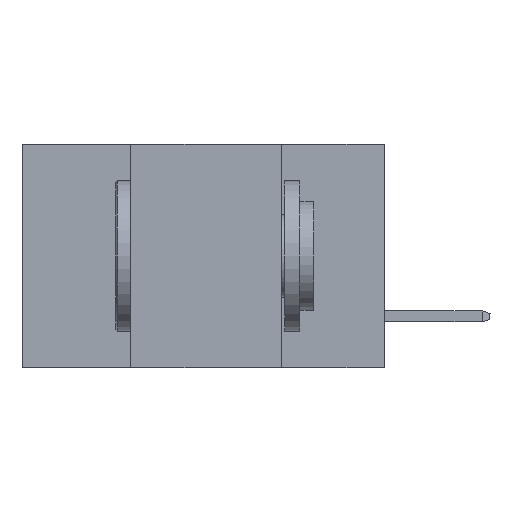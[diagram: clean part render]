
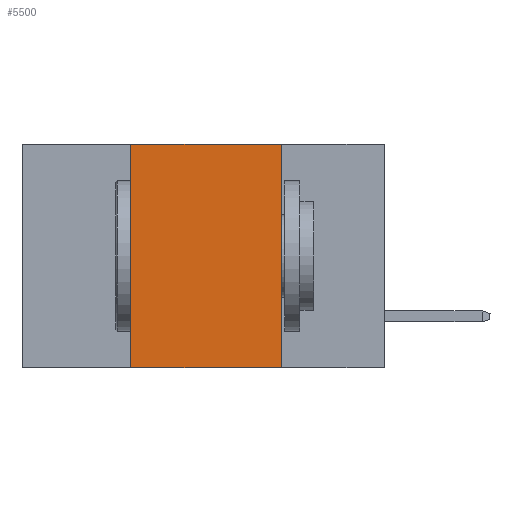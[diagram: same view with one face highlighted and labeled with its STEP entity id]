
A CAD part, left-side view. The second image highlights one B-rep face of the part: STEP entity #5500.
In plain terms, the highlighted planar face has unit normal (-1, 0, 0).
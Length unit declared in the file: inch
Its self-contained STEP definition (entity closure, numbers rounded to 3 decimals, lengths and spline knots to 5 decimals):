
#120 = VECTOR ( 'NONE', #9460, 39.37008 ) ;
#248 = ORIENTED_EDGE ( 'NONE', *, *, #519, .F. ) ;
#519 = EDGE_CURVE ( 'NONE', #4110, #1540, #8587, .T. ) ;
#628 = VECTOR ( 'NONE', #6161, 39.37008 ) ;
#890 = VECTOR ( 'NONE', #1525, 39.37008 ) ;
#1060 = CARTESIAN_POINT ( 'NONE',  ( 0., 0.6, 0. ) ) ;
#1525 = DIRECTION ( 'NONE',  ( 0., -1., 0. ) ) ;
#1540 = VERTEX_POINT ( 'NONE', #7640 ) ;
#2451 = LINE ( 'NONE', #4931, #2628 ) ;
#2628 = VECTOR ( 'NONE', #7295, 39.37008 ) ;
#3662 = DIRECTION ( 'NONE',  ( 1., 0., 0. ) ) ;
#3677 = CARTESIAN_POINT ( 'NONE',  ( 0., 0.6, 0. ) ) ;
#3754 = LINE ( 'NONE', #6472, #120 ) ;
#4110 = VERTEX_POINT ( 'NONE', #8126 ) ;
#4931 = CARTESIAN_POINT ( 'NONE',  ( 0., 0.42, -0.37 ) ) ;
#5342 = ORIENTED_EDGE ( 'NONE', *, *, #6249, .F. ) ;
#5350 = ORIENTED_EDGE ( 'NONE', *, *, #9890, .F. ) ;
#5378 = AXIS2_PLACEMENT_3D ( 'NONE', #1060, #3662, #6031 ) ;
#5500 = ADVANCED_FACE ( 'NONE', ( #9274 ), #7701, .F. ) ;
#5789 = EDGE_CURVE ( 'NONE', #8296, #7349, #6609, .T. ) ;
#6031 = DIRECTION ( 'NONE',  ( 0., 0., -1. ) ) ;
#6069 = CARTESIAN_POINT ( 'NONE',  ( 0., 0.17, -0.37 ) ) ;
#6161 = DIRECTION ( 'NONE',  ( 0., -1., 0. ) ) ;
#6249 = EDGE_CURVE ( 'NONE', #8296, #4110, #2451, .T. ) ;
#6472 = CARTESIAN_POINT ( 'NONE',  ( 0., 0.17, -0.37 ) ) ;
#6609 = LINE ( 'NONE', #8119, #890 ) ;
#7295 = DIRECTION ( 'NONE',  ( 0., 0., 1. ) ) ;
#7349 = VERTEX_POINT ( 'NONE', #6069 ) ;
#7640 = CARTESIAN_POINT ( 'NONE',  ( 0., 0.17, 0. ) ) ;
#7701 = PLANE ( 'NONE',  #5378 ) ;
#8119 = CARTESIAN_POINT ( 'NONE',  ( 0., 0.6, -0.37 ) ) ;
#8126 = CARTESIAN_POINT ( 'NONE',  ( 0., 0.42, 0. ) ) ;
#8296 = VERTEX_POINT ( 'NONE', #9604 ) ;
#8587 = LINE ( 'NONE', #3677, #628 ) ;
#9274 = FACE_OUTER_BOUND ( 'NONE', #10531, .T. ) ;
#9460 = DIRECTION ( 'NONE',  ( 0., 0., -1. ) ) ;
#9604 = CARTESIAN_POINT ( 'NONE',  ( 0., 0.42, -0.37 ) ) ;
#9890 = EDGE_CURVE ( 'NONE', #1540, #7349, #3754, .T. ) ;
#9981 = ORIENTED_EDGE ( 'NONE', *, *, #5789, .T. ) ;
#10531 = EDGE_LOOP ( 'NONE', ( #5350, #248, #5342, #9981 ) ) ;
